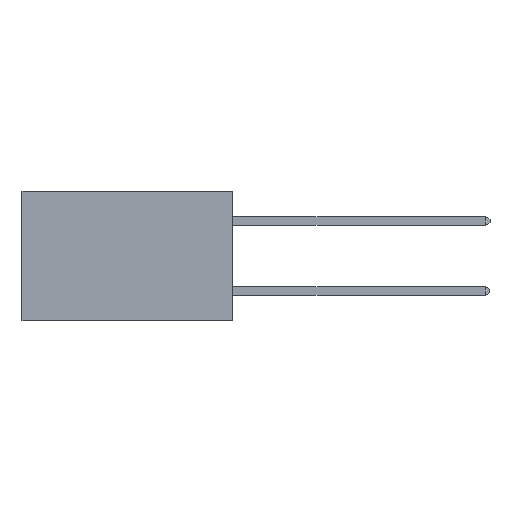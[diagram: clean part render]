
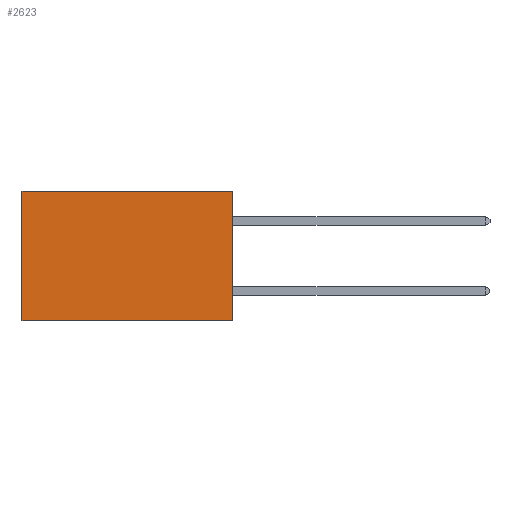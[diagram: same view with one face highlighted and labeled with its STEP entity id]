
A CAD part, left-side view. The second image highlights one B-rep face of the part: STEP entity #2623.
In plain terms, the highlighted planar face has unit normal (-1, 0, 0).
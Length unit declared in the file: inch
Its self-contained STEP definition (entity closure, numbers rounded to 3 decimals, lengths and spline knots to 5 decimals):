
#127 = DIRECTION ( 'NONE',  ( 0., 0., -1. ) ) ;
#252 = DIRECTION ( 'NONE',  ( 0., 1., 0. ) ) ;
#716 = CARTESIAN_POINT ( 'NONE',  ( 0.2875, 0., 0. ) ) ;
#1233 = LINE ( 'NONE', #716, #9993 ) ;
#1337 = CARTESIAN_POINT ( 'NONE',  ( 0.2875, 0.6, -0.37 ) ) ;
#2164 = LINE ( 'NONE', #20719, #14914 ) ;
#2431 = VERTEX_POINT ( 'NONE', #16007 ) ;
#2623 = ADVANCED_FACE ( 'NONE', ( #4125 ), #6195, .F. ) ;
#2806 = ORIENTED_EDGE ( 'NONE', *, *, #18144, .F. ) ;
#2812 = VERTEX_POINT ( 'NONE', #1337 ) ;
#3937 = AXIS2_PLACEMENT_3D ( 'NONE', #4412, #7850, #7928 ) ;
#4125 = FACE_OUTER_BOUND ( 'NONE', #9164, .T. ) ;
#4412 = CARTESIAN_POINT ( 'NONE',  ( 0.2875, 0., 0. ) ) ;
#4553 = LINE ( 'NONE', #20831, #21988 ) ;
#4908 = VERTEX_POINT ( 'NONE', #21683 ) ;
#6195 = PLANE ( 'NONE',  #3937 ) ;
#6552 = CARTESIAN_POINT ( 'NONE',  ( 0.2875, 0., 0. ) ) ;
#7850 = DIRECTION ( 'NONE',  ( 1., 0., 0. ) ) ;
#7928 = DIRECTION ( 'NONE',  ( 0., 0., -1. ) ) ;
#8290 = DIRECTION ( 'NONE',  ( 0., 1., 0. ) ) ;
#9164 = EDGE_LOOP ( 'NONE', ( #17131, #2806, #19970, #19516 ) ) ;
#9475 = DIRECTION ( 'NONE',  ( 0., 0., -1. ) ) ;
#9993 = VECTOR ( 'NONE', #9475, 39.37008 ) ;
#10822 = VECTOR ( 'NONE', #8290, 39.37008 ) ;
#10999 = CARTESIAN_POINT ( 'NONE',  ( 0.2875, 0., -0.37 ) ) ;
#12614 = VERTEX_POINT ( 'NONE', #10999 ) ;
#14914 = VECTOR ( 'NONE', #127, 39.37008 ) ;
#15743 = EDGE_CURVE ( 'NONE', #2431, #2812, #2164, .T. ) ;
#16007 = CARTESIAN_POINT ( 'NONE',  ( 0.2875, 0.6, 0. ) ) ;
#17018 = EDGE_CURVE ( 'NONE', #4908, #12614, #1233, .T. ) ;
#17131 = ORIENTED_EDGE ( 'NONE', *, *, #15743, .T. ) ;
#18144 = EDGE_CURVE ( 'NONE', #12614, #2812, #4553, .T. ) ;
#19516 = ORIENTED_EDGE ( 'NONE', *, *, #21084, .T. ) ;
#19830 = LINE ( 'NONE', #6552, #10822 ) ;
#19970 = ORIENTED_EDGE ( 'NONE', *, *, #17018, .F. ) ;
#20719 = CARTESIAN_POINT ( 'NONE',  ( 0.2875, 0.6, 0. ) ) ;
#20831 = CARTESIAN_POINT ( 'NONE',  ( 0.2875, 0., -0.37 ) ) ;
#21084 = EDGE_CURVE ( 'NONE', #4908, #2431, #19830, .T. ) ;
#21683 = CARTESIAN_POINT ( 'NONE',  ( 0.2875, 0., 0. ) ) ;
#21988 = VECTOR ( 'NONE', #252, 39.37008 ) ;
